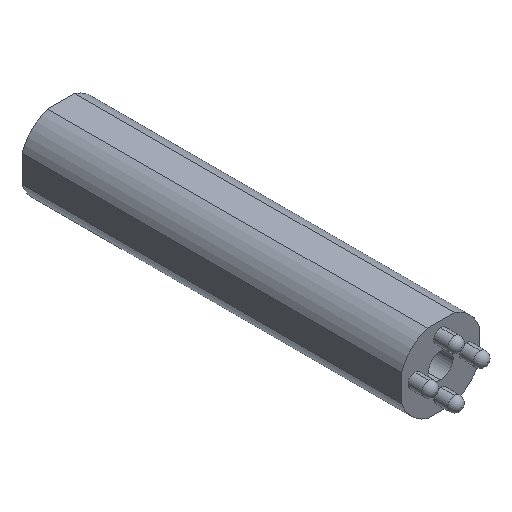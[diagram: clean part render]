
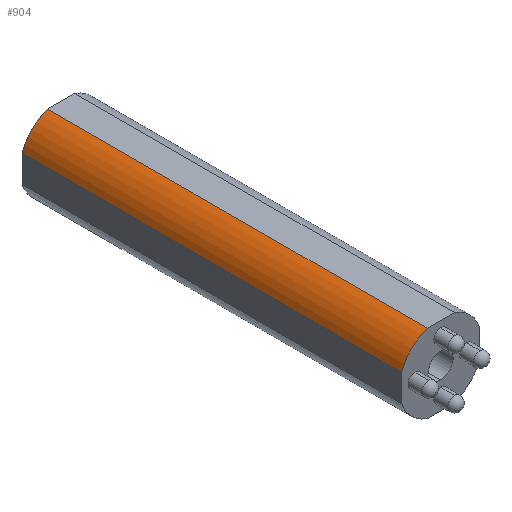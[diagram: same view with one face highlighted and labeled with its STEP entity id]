
A CAD part, isometric view. The second image highlights one B-rep face of the part: STEP entity #904.
In plain terms, the highlighted cylindrical face has radius 15.243 mm (diameter 30.485 mm), a partial arc.
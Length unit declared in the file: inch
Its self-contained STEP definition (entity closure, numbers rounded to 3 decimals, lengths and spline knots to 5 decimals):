
#46 = DIRECTION ( 'NONE',  ( 0., -1., 0. ) ) ;
#48 = LINE ( 'NONE', #60, #1104 ) ;
#49 = DIRECTION ( 'NONE',  ( 0., -1., 0. ) ) ;
#51 = CARTESIAN_POINT ( 'NONE',  ( 0.37035, 5.5, 0.37035 ) ) ;
#56 = LINE ( 'NONE', #51, #1100 ) ;
#60 = CARTESIAN_POINT ( 'NONE',  ( -0.00056, 5.5, 0. ) ) ;
#68 = DIRECTION ( 'NONE',  ( 0., -1., 0. ) ) ;
#71 = DIRECTION ( 'NONE',  ( 0., 0., -1. ) ) ;
#92 = CARTESIAN_POINT ( 'NONE',  ( 0.56634, 5.5, -0.19685 ) ) ;
#201 = CARTESIAN_POINT ( 'NONE',  ( 0.56634, 5.5, -0.19685 ) ) ;
#212 = DIRECTION ( 'NONE',  ( 0., 1., 0. ) ) ;
#216 = DIRECTION ( 'NONE',  ( 0., 0., 1. ) ) ;
#254 = EDGE_LOOP ( 'NONE', ( #734, #730, #729, #721 ) ) ;
#319 = CARTESIAN_POINT ( 'NONE',  ( 0.37035, 5.5, 0.37035 ) ) ;
#332 = CARTESIAN_POINT ( 'NONE',  ( -0.00056, 0., 0. ) ) ;
#337 = CARTESIAN_POINT ( 'NONE',  ( -0.00056, 5.5, 0. ) ) ;
#342 = CARTESIAN_POINT ( 'NONE',  ( 0.37035, 0., 0.37035 ) ) ;
#392 = CARTESIAN_POINT ( 'NONE',  ( 0.56634, 0., -0.19685 ) ) ;
#393 = DIRECTION ( 'NONE',  ( 0., 1., 0. ) ) ;
#441 = DIRECTION ( 'NONE',  ( 0., 0., 1. ) ) ;
#683 = VERTEX_POINT ( 'NONE', #332 ) ;
#691 = VERTEX_POINT ( 'NONE', #337 ) ;
#695 = VERTEX_POINT ( 'NONE', #342 ) ;
#715 = VERTEX_POINT ( 'NONE', #319 ) ;
#721 = ORIENTED_EDGE ( 'NONE', *, *, #893, .T. ) ;
#729 = ORIENTED_EDGE ( 'NONE', *, *, #874, .F. ) ;
#730 = ORIENTED_EDGE ( 'NONE', *, *, #891, .F. ) ;
#734 = ORIENTED_EDGE ( 'NONE', *, *, #812, .T. ) ;
#812 = EDGE_CURVE ( 'NONE', #683, #695, #946, .T. ) ;
#874 = EDGE_CURVE ( 'NONE', #691, #715, #927, .T. ) ;
#891 = EDGE_CURVE ( 'NONE', #715, #695, #56, .T. ) ;
#893 = EDGE_CURVE ( 'NONE', #691, #683, #48, .T. ) ;
#904 = ADVANCED_FACE ( 'NONE', ( #1107 ), #1112, .T. ) ;
#927 = CIRCLE ( 'NONE', #1077, 0.60011 ) ;
#946 = CIRCLE ( 'NONE', #999, 0.60011 ) ;
#999 = AXIS2_PLACEMENT_3D ( 'NONE', #392, #393, #441 ) ;
#1077 = AXIS2_PLACEMENT_3D ( 'NONE', #201, #212, #216 ) ;
#1100 = VECTOR ( 'NONE', #49, 39.37008 ) ;
#1104 = VECTOR ( 'NONE', #46, 39.37008 ) ;
#1107 = FACE_OUTER_BOUND ( 'NONE', #254, .T. ) ;
#1112 = CYLINDRICAL_SURFACE ( 'NONE', #1117, 0.60011 ) ;
#1117 = AXIS2_PLACEMENT_3D ( 'NONE', #92, #68, #71 ) ;
